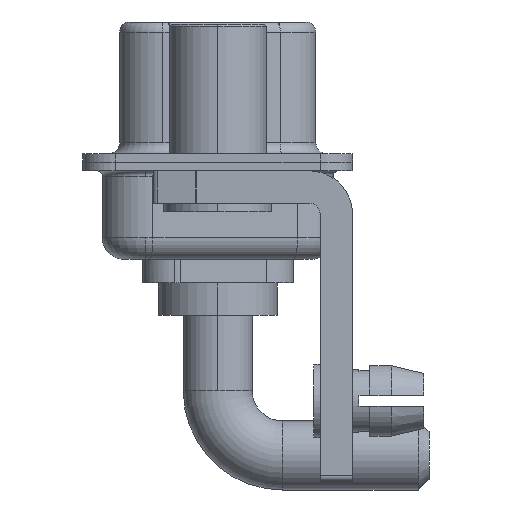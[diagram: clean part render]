
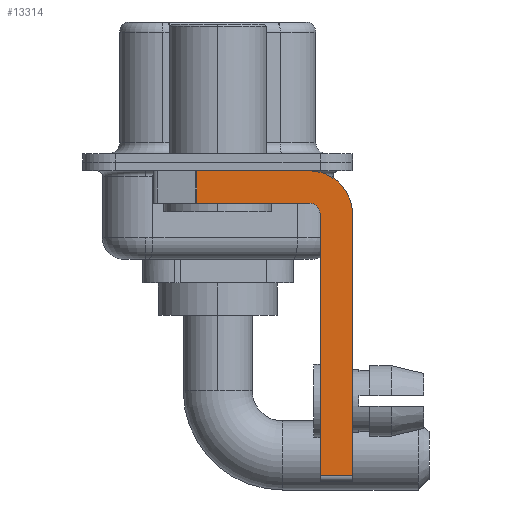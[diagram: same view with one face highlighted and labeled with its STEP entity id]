
A CAD part, left-side view. The second image highlights one B-rep face of the part: STEP entity #13314.
In plain terms, the highlighted planar face has unit normal (-1, 0, 0).
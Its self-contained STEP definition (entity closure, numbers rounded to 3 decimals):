
#269 = ORIENTED_EDGE ( 'NONE', *, *, #5808, .F. ) ;
#384 = VECTOR ( 'NONE', #13841, 1000. ) ;
#505 = EDGE_CURVE ( 'NONE', #12511, #16154, #18313, .T. ) ;
#642 = CARTESIAN_POINT ( 'NONE',  ( -2.9, -4.75, -14.55 ) ) ;
#815 = DIRECTION ( 'NONE',  ( 1., 0., 0. ) ) ;
#1022 = CARTESIAN_POINT ( 'NONE',  ( -2.9, -4.25, -2.4 ) ) ;
#1027 = CARTESIAN_POINT ( 'NONE',  ( -2.9, -6.25, -2.4 ) ) ;
#1724 = CARTESIAN_POINT ( 'NONE',  ( -2.9, 0.978, -1.9 ) ) ;
#2014 = DIRECTION ( 'NONE',  ( 0., 0., -1. ) ) ;
#2415 = VECTOR ( 'NONE', #2014, 1000. ) ;
#2514 = CARTESIAN_POINT ( 'NONE',  ( -2.9, 0.978, -1.9 ) ) ;
#3039 = DIRECTION ( 'NONE',  ( 0., 0., 1. ) ) ;
#3335 = ORIENTED_EDGE ( 'NONE', *, *, #14834, .F. ) ;
#3456 = VECTOR ( 'NONE', #3039, 1000. ) ;
#3594 = DIRECTION ( 'NONE',  ( 0., 0., -1. ) ) ;
#3733 = AXIS2_PLACEMENT_3D ( 'NONE', #17200, #14194, #3594 ) ;
#4036 = CARTESIAN_POINT ( 'NONE',  ( -2.9, -4.25, -14.55 ) ) ;
#4895 = EDGE_CURVE ( 'NONE', #15505, #9647, #7602, .T. ) ;
#5338 = DIRECTION ( 'NONE',  ( -1., 0., 0. ) ) ;
#5429 = VERTEX_POINT ( 'NONE', #1027 ) ;
#5808 = EDGE_CURVE ( 'NONE', #17555, #16154, #9644, .T. ) ;
#5944 = VERTEX_POINT ( 'NONE', #17792 ) ;
#6298 = LINE ( 'NONE', #9364, #16628 ) ;
#6300 = DIRECTION ( 'NONE',  ( 0., -1., 0. ) ) ;
#6873 = DIRECTION ( 'NONE',  ( 0., 0., -1. ) ) ;
#7022 = EDGE_LOOP ( 'NONE', ( #15162, #18434, #269, #15892, #14112, #8631, #13285, #3335 ) ) ;
#7151 = CARTESIAN_POINT ( 'NONE',  ( -2.9, -6.25, -14.55 ) ) ;
#7602 = LINE ( 'NONE', #13651, #3456 ) ;
#7988 = CARTESIAN_POINT ( 'NONE',  ( -2.9, 0.978, -0.4 ) ) ;
#8076 = DIRECTION ( 'NONE',  ( 0., 0., -1. ) ) ;
#8513 = EDGE_CURVE ( 'NONE', #12511, #5944, #9571, .T. ) ;
#8625 = DIRECTION ( 'NONE',  ( 0., 0., 1. ) ) ;
#8631 = ORIENTED_EDGE ( 'NONE', *, *, #15756, .T. ) ;
#9364 = CARTESIAN_POINT ( 'NONE',  ( -2.9, -6.25, -2.4 ) ) ;
#9571 = LINE ( 'NONE', #12646, #384 ) ;
#9644 = LINE ( 'NONE', #15710, #19018 ) ;
#9647 = VERTEX_POINT ( 'NONE', #15232 ) ;
#9812 = CARTESIAN_POINT ( 'NONE',  ( -2.9, -4.25, -2.4 ) ) ;
#9834 = EDGE_CURVE ( 'NONE', #5429, #18628, #6298, .T. ) ;
#11132 = PLANE ( 'NONE',  #3733 ) ;
#12295 = CARTESIAN_POINT ( 'NONE',  ( -2.9, -4.25, -1.9 ) ) ;
#12511 = VERTEX_POINT ( 'NONE', #7988 ) ;
#12646 = CARTESIAN_POINT ( 'NONE',  ( -2.9, 3., -0.4 ) ) ;
#13285 = ORIENTED_EDGE ( 'NONE', *, *, #9834, .F. ) ;
#13314 = ADVANCED_FACE ( 'NONE', ( #18674 ), #11132, .F. ) ;
#13651 = CARTESIAN_POINT ( 'NONE',  ( -2.9, -4.75, -14.8 ) ) ;
#13841 = DIRECTION ( 'NONE',  ( 0., -1., 0. ) ) ;
#13868 = CIRCLE ( 'NONE', #19267, 2. ) ;
#14112 = ORIENTED_EDGE ( 'NONE', *, *, #4895, .F. ) ;
#14194 = DIRECTION ( 'NONE',  ( 1., 0., 0. ) ) ;
#14834 = EDGE_CURVE ( 'NONE', #5944, #5429, #13868, .T. ) ;
#15162 = ORIENTED_EDGE ( 'NONE', *, *, #8513, .F. ) ;
#15232 = CARTESIAN_POINT ( 'NONE',  ( -2.9, -4.75, -2.4 ) ) ;
#15409 = DIRECTION ( 'NONE',  ( 0., 1., 0. ) ) ;
#15505 = VERTEX_POINT ( 'NONE', #642 ) ;
#15541 = CIRCLE ( 'NONE', #16498, 0.5 ) ;
#15710 = CARTESIAN_POINT ( 'NONE',  ( -2.9, -4.25, -1.9 ) ) ;
#15756 = EDGE_CURVE ( 'NONE', #15505, #18628, #17642, .T. ) ;
#15892 = ORIENTED_EDGE ( 'NONE', *, *, #16995, .F. ) ;
#16154 = VERTEX_POINT ( 'NONE', #2514 ) ;
#16498 = AXIS2_PLACEMENT_3D ( 'NONE', #9812, #5338, #8625 ) ;
#16628 = VECTOR ( 'NONE', #8076, 1000. ) ;
#16995 = EDGE_CURVE ( 'NONE', #9647, #17555, #15541, .T. ) ;
#17200 = CARTESIAN_POINT ( 'NONE',  ( -2.9, -4.25, -2.4 ) ) ;
#17405 = VECTOR ( 'NONE', #6300, 1000. ) ;
#17555 = VERTEX_POINT ( 'NONE', #12295 ) ;
#17642 = LINE ( 'NONE', #4036, #17405 ) ;
#17792 = CARTESIAN_POINT ( 'NONE',  ( -2.9, -4.25, -0.4 ) ) ;
#18313 = LINE ( 'NONE', #1724, #2415 ) ;
#18434 = ORIENTED_EDGE ( 'NONE', *, *, #505, .T. ) ;
#18628 = VERTEX_POINT ( 'NONE', #7151 ) ;
#18674 = FACE_OUTER_BOUND ( 'NONE', #7022, .T. ) ;
#19018 = VECTOR ( 'NONE', #15409, 1000. ) ;
#19267 = AXIS2_PLACEMENT_3D ( 'NONE', #1022, #815, #6873 ) ;
